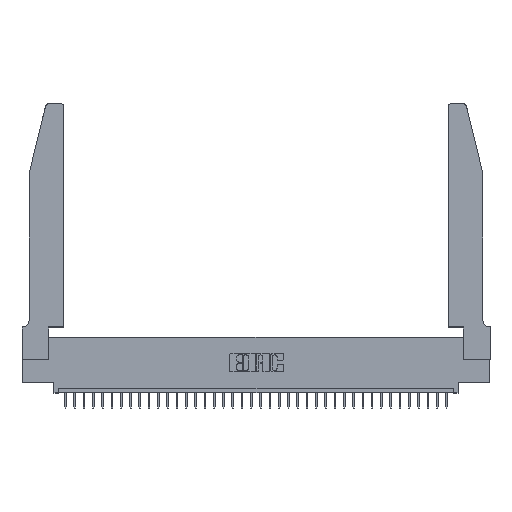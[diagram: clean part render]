
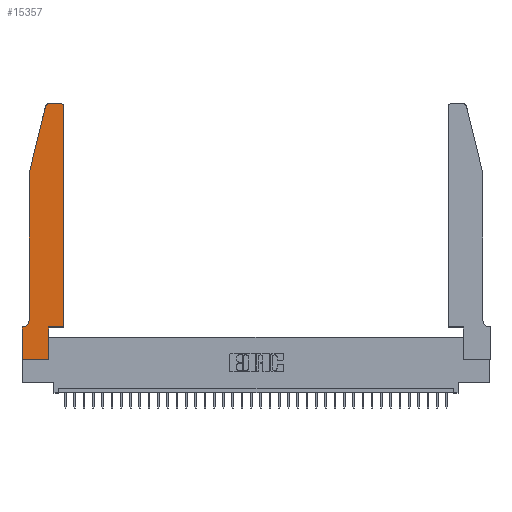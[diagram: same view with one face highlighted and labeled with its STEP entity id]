
A CAD part, top view. The second image highlights one B-rep face of the part: STEP entity #15357.
In plain terms, the highlighted planar face has unit normal (0, 0, 1).
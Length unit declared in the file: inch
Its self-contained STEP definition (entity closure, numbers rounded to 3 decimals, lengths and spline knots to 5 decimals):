
#467 = DIRECTION ( 'NONE',  ( 0., 0., 1. ) ) ;
#658 = DIRECTION ( 'NONE',  ( 1., 0., 0. ) ) ;
#919 = CARTESIAN_POINT ( 'NONE',  ( 0.4505, 0.35, 0.37 ) ) ;
#1295 = CARTESIAN_POINT ( 'NONE',  ( 0.0755, 2., 0.37 ) ) ;
#2157 = CARTESIAN_POINT ( 'NONE',  ( 0.0755, 0.35, 0.37 ) ) ;
#2492 = LINE ( 'NONE', #8163, #32553 ) ;
#3283 = VECTOR ( 'NONE', #27843, 39.37008 ) ;
#3646 = VERTEX_POINT ( 'NONE', #9756 ) ;
#4021 = VERTEX_POINT ( 'NONE', #26947 ) ;
#4177 = VERTEX_POINT ( 'NONE', #27036 ) ;
#5182 = LINE ( 'NONE', #2157, #28199 ) ;
#7288 = FACE_OUTER_BOUND ( 'NONE', #28944, .T. ) ;
#7688 = CARTESIAN_POINT ( 'NONE',  ( 0.284, 2.72, 0.37 ) ) ;
#7998 = CARTESIAN_POINT ( 'NONE',  ( 0., 0.35, 0.37 ) ) ;
#8142 = CARTESIAN_POINT ( 'NONE',  ( 0., 0., 0.37 ) ) ;
#8163 = CARTESIAN_POINT ( 'NONE',  ( 0., 0., 0.37 ) ) ;
#8197 = EDGE_CURVE ( 'NONE', #3646, #4177, #20093, .T. ) ;
#8686 = VERTEX_POINT ( 'NONE', #31685 ) ;
#8858 = DIRECTION ( 'NONE',  ( -1., 0., 0. ) ) ;
#8941 = CARTESIAN_POINT ( 'NONE',  ( 0.4205, 2.75, 0.37 ) ) ;
#9116 = VERTEX_POINT ( 'NONE', #8142 ) ;
#9276 = EDGE_CURVE ( 'NONE', #4021, #13756, #23166, .T. ) ;
#9756 = CARTESIAN_POINT ( 'NONE',  ( 0.2865, 0., 0.37 ) ) ;
#10334 = CIRCLE ( 'NONE', #12643, 0.03 ) ;
#10631 = EDGE_CURVE ( 'NONE', #18041, #8686, #35461, .T. ) ;
#10869 = DIRECTION ( 'NONE',  ( 1., 0., 0. ) ) ;
#10928 = DIRECTION ( 'NONE',  ( -1., 0., 0. ) ) ;
#10956 = VERTEX_POINT ( 'NONE', #27664 ) ;
#11117 = ORIENTED_EDGE ( 'NONE', *, *, #10631, .T. ) ;
#11213 = VERTEX_POINT ( 'NONE', #17109 ) ;
#11229 = ORIENTED_EDGE ( 'NONE', *, *, #19309, .T. ) ;
#11355 = LINE ( 'NONE', #12075, #29928 ) ;
#11417 = CARTESIAN_POINT ( 'NONE',  ( 0.2865, 0.35, 0.37 ) ) ;
#11493 = ORIENTED_EDGE ( 'NONE', *, *, #20316, .T. ) ;
#11961 = EDGE_CURVE ( 'NONE', #4177, #18220, #14165, .T. ) ;
#12075 = CARTESIAN_POINT ( 'NONE',  ( 0.2605, 2.75, 0.37 ) ) ;
#12435 = VECTOR ( 'NONE', #658, 39.37008 ) ;
#12643 = AXIS2_PLACEMENT_3D ( 'NONE', #7688, #21559, #24365 ) ;
#13756 = VERTEX_POINT ( 'NONE', #8941 ) ;
#13936 = DIRECTION ( 'NONE',  ( 0., -1., 0. ) ) ;
#14165 = LINE ( 'NONE', #14945, #12435 ) ;
#14457 = ORIENTED_EDGE ( 'NONE', *, *, #8197, .T. ) ;
#14486 = ORIENTED_EDGE ( 'NONE', *, *, #18491, .T. ) ;
#14798 = EDGE_CURVE ( 'NONE', #25303, #9116, #2492, .T. ) ;
#14945 = CARTESIAN_POINT ( 'NONE',  ( 0.4505, 0.35, 0.37 ) ) ;
#15224 = LINE ( 'NONE', #32094, #20578 ) ;
#15357 = ADVANCED_FACE ( 'NONE', ( #7288 ), #22342, .T. ) ;
#15517 = DIRECTION ( 'NONE',  ( 0., 0., -1. ) ) ;
#16088 = EDGE_CURVE ( 'NONE', #28460, #18041, #19178, .T. ) ;
#16977 = CIRCLE ( 'NONE', #24386, 0.07 ) ;
#17109 = CARTESIAN_POINT ( 'NONE',  ( 0.0055, 0.35, 0.37 ) ) ;
#17138 = CARTESIAN_POINT ( 'NONE',  ( 0.4505, 0.35, 0.37 ) ) ;
#17357 = CARTESIAN_POINT ( 'NONE',  ( 0.4205, 2.72, 0.37 ) ) ;
#17931 = ORIENTED_EDGE ( 'NONE', *, *, #14798, .T. ) ;
#17954 = CARTESIAN_POINT ( 'NONE',  ( 0.25487, 2.72718, 0.37 ) ) ;
#18041 = VERTEX_POINT ( 'NONE', #23160 ) ;
#18196 = ORIENTED_EDGE ( 'NONE', *, *, #25119, .T. ) ;
#18220 = VERTEX_POINT ( 'NONE', #919 ) ;
#18491 = EDGE_CURVE ( 'NONE', #11213, #25303, #5182, .T. ) ;
#19178 = LINE ( 'NONE', #31538, #24899 ) ;
#19309 = EDGE_CURVE ( 'NONE', #13756, #10956, #11355, .T. ) ;
#20093 = LINE ( 'NONE', #11417, #3283 ) ;
#20221 = DIRECTION ( 'NONE',  ( 1., 0., 0. ) ) ;
#20316 = EDGE_CURVE ( 'NONE', #8686, #11213, #16977, .T. ) ;
#20578 = VECTOR ( 'NONE', #26638, 39.37008 ) ;
#21131 = CARTESIAN_POINT ( 'NONE',  ( 0.0055, 0.42, 0.37 ) ) ;
#21535 = ORIENTED_EDGE ( 'NONE', *, *, #29341, .T. ) ;
#21559 = DIRECTION ( 'NONE',  ( 0., 0., 1. ) ) ;
#21785 = VECTOR ( 'NONE', #25798, 39.37008 ) ;
#22342 = PLANE ( 'NONE',  #30936 ) ;
#23160 = CARTESIAN_POINT ( 'NONE',  ( 0.0755, 2., 0.37 ) ) ;
#23166 = CIRCLE ( 'NONE', #30512, 0.03 ) ;
#24365 = DIRECTION ( 'NONE',  ( 1., 0., 0. ) ) ;
#24386 = AXIS2_PLACEMENT_3D ( 'NONE', #21131, #15517, #26908 ) ;
#24848 = EDGE_CURVE ( 'NONE', #10956, #28460, #10334, .T. ) ;
#24899 = VECTOR ( 'NONE', #25829, 39.37008 ) ;
#25119 = EDGE_CURVE ( 'NONE', #18220, #4021, #29714, .T. ) ;
#25303 = VERTEX_POINT ( 'NONE', #29006 ) ;
#25798 = DIRECTION ( 'NONE',  ( 0., 1., 0. ) ) ;
#25829 = DIRECTION ( 'NONE',  ( -0.239, -0.971, 0. ) ) ;
#26638 = DIRECTION ( 'NONE',  ( 1., 0., 0. ) ) ;
#26847 = DIRECTION ( 'NONE',  ( 0., -1., 0. ) ) ;
#26908 = DIRECTION ( 'NONE',  ( -1., 0., 0. ) ) ;
#26947 = CARTESIAN_POINT ( 'NONE',  ( 0.4505, 2.72, 0.37 ) ) ;
#27036 = CARTESIAN_POINT ( 'NONE',  ( 0.2865, 0.35, 0.37 ) ) ;
#27664 = CARTESIAN_POINT ( 'NONE',  ( 0.284, 2.75, 0.37 ) ) ;
#27763 = DIRECTION ( 'NONE',  ( 0., 0., 1. ) ) ;
#27843 = DIRECTION ( 'NONE',  ( 0., 1., 0. ) ) ;
#28199 = VECTOR ( 'NONE', #10928, 39.37008 ) ;
#28460 = VERTEX_POINT ( 'NONE', #17954 ) ;
#28944 = EDGE_LOOP ( 'NONE', ( #11229, #32419, #29632, #11117, #11493, #14486, #17931, #21535, #14457, #30520, #18196, #32383 ) ) ;
#29006 = CARTESIAN_POINT ( 'NONE',  ( 0., 0.35, 0.37 ) ) ;
#29341 = EDGE_CURVE ( 'NONE', #9116, #3646, #15224, .T. ) ;
#29632 = ORIENTED_EDGE ( 'NONE', *, *, #16088, .T. ) ;
#29714 = LINE ( 'NONE', #17138, #21785 ) ;
#29928 = VECTOR ( 'NONE', #8858, 39.37008 ) ;
#30512 = AXIS2_PLACEMENT_3D ( 'NONE', #17357, #467, #20221 ) ;
#30520 = ORIENTED_EDGE ( 'NONE', *, *, #11961, .T. ) ;
#30936 = AXIS2_PLACEMENT_3D ( 'NONE', #7998, #27763, #10869 ) ;
#31477 = VECTOR ( 'NONE', #26847, 39.37008 ) ;
#31538 = CARTESIAN_POINT ( 'NONE',  ( 0.0755, 2., 0.37 ) ) ;
#31685 = CARTESIAN_POINT ( 'NONE',  ( 0.0755, 0.42, 0.37 ) ) ;
#32094 = CARTESIAN_POINT ( 'NONE',  ( 0., 0., 0.37 ) ) ;
#32383 = ORIENTED_EDGE ( 'NONE', *, *, #9276, .T. ) ;
#32419 = ORIENTED_EDGE ( 'NONE', *, *, #24848, .T. ) ;
#32553 = VECTOR ( 'NONE', #13936, 39.37008 ) ;
#35461 = LINE ( 'NONE', #1295, #31477 ) ;
